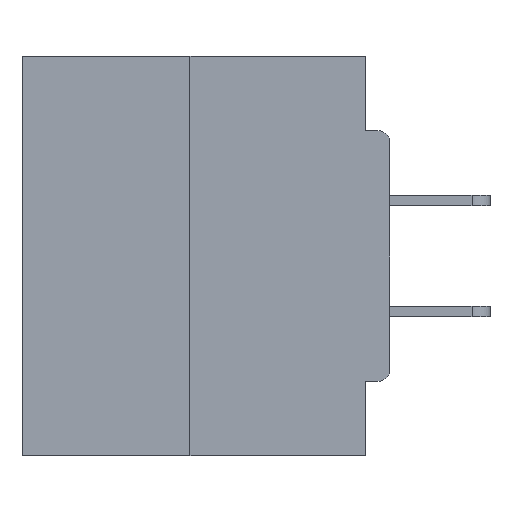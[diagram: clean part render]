
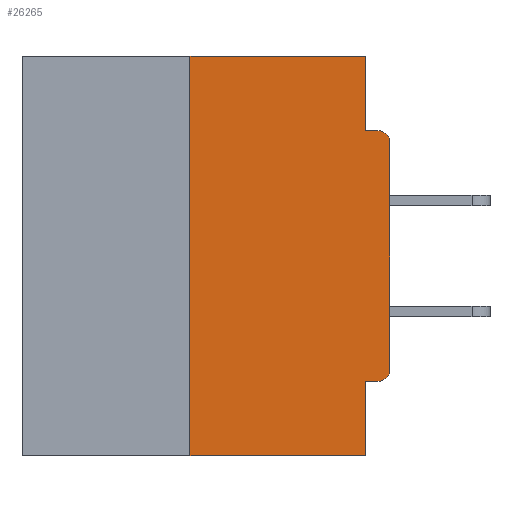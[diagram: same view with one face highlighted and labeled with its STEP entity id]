
A CAD part, left-side view. The second image highlights one B-rep face of the part: STEP entity #26265.
In plain terms, the highlighted planar face has unit normal (-1, 0, 0).
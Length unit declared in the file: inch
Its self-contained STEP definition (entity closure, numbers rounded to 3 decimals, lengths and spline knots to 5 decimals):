
#875 = DIRECTION ( 'NONE',  ( 0., 1., 0. ) ) ;
#1346 = CARTESIAN_POINT ( 'NONE',  ( 0., 0.46, 0. ) ) ;
#1678 = CARTESIAN_POINT ( 'NONE',  ( 0., 0.031, 0. ) ) ;
#2072 = DIRECTION ( 'NONE',  ( 0., 0., -1. ) ) ;
#2079 = AXIS2_PLACEMENT_3D ( 'NONE', #20776, #26328, #14355 ) ;
#2173 = CARTESIAN_POINT ( 'NONE',  ( 0., 0.031, -0.0935 ) ) ;
#2442 = CIRCLE ( 'NONE', #2079, 0.015 ) ;
#2732 = ORIENTED_EDGE ( 'NONE', *, *, #28134, .T. ) ;
#3569 = LINE ( 'NONE', #17001, #16551 ) ;
#4416 = VERTEX_POINT ( 'NONE', #1678 ) ;
#4546 = FACE_OUTER_BOUND ( 'NONE', #31437, .T. ) ;
#4741 = ORIENTED_EDGE ( 'NONE', *, *, #11772, .T. ) ;
#5494 = AXIS2_PLACEMENT_3D ( 'NONE', #18120, #24170, #39622 ) ;
#5855 = CARTESIAN_POINT ( 'NONE',  ( 0., 0., 0. ) ) ;
#6552 = LINE ( 'NONE', #32790, #29176 ) ;
#7020 = VECTOR ( 'NONE', #16874, 39.37008 ) ;
#7165 = CARTESIAN_POINT ( 'NONE',  ( 0., 0.25, 0. ) ) ;
#7606 = EDGE_CURVE ( 'NONE', #38162, #8715, #23775, .T. ) ;
#7782 = CARTESIAN_POINT ( 'NONE',  ( 0., 0.015, -0.0935 ) ) ;
#8039 = DIRECTION ( 'NONE',  ( 0., -1., 0. ) ) ;
#8715 = VERTEX_POINT ( 'NONE', #27837 ) ;
#8838 = ORIENTED_EDGE ( 'NONE', *, *, #26381, .F. ) ;
#9383 = ORIENTED_EDGE ( 'NONE', *, *, #21197, .T. ) ;
#10501 = ORIENTED_EDGE ( 'NONE', *, *, #39046, .F. ) ;
#11159 = VERTEX_POINT ( 'NONE', #16695 ) ;
#11772 = EDGE_CURVE ( 'NONE', #11159, #28743, #6552, .T. ) ;
#13876 = PLANE ( 'NONE',  #21875 ) ;
#13897 = CARTESIAN_POINT ( 'NONE',  ( 0., 0., -0.1085 ) ) ;
#14192 = CARTESIAN_POINT ( 'NONE',  ( 0., 0., -0.3915 ) ) ;
#14355 = DIRECTION ( 'NONE',  ( 0., 0., -1. ) ) ;
#15126 = EDGE_CURVE ( 'NONE', #16655, #4416, #16338, .T. ) ;
#16338 = LINE ( 'NONE', #36605, #36119 ) ;
#16551 = VECTOR ( 'NONE', #2072, 39.37008 ) ;
#16650 = DIRECTION ( 'NONE',  ( 1., 0., 0. ) ) ;
#16655 = VERTEX_POINT ( 'NONE', #23338 ) ;
#16695 = CARTESIAN_POINT ( 'NONE',  ( 0., 0.25, -0.5 ) ) ;
#16832 = ORIENTED_EDGE ( 'NONE', *, *, #23366, .F. ) ;
#16874 = DIRECTION ( 'NONE',  ( 0., 0., -1. ) ) ;
#16960 = VERTEX_POINT ( 'NONE', #13897 ) ;
#17001 = CARTESIAN_POINT ( 'NONE',  ( 0., 0.031, -0.5 ) ) ;
#17067 = DIRECTION ( 'NONE',  ( 0., 0., -1. ) ) ;
#17168 = ORIENTED_EDGE ( 'NONE', *, *, #15126, .F. ) ;
#18120 = CARTESIAN_POINT ( 'NONE',  ( 0., 0.015, -0.1085 ) ) ;
#20385 = CIRCLE ( 'NONE', #5494, 0.015 ) ;
#20776 = CARTESIAN_POINT ( 'NONE',  ( 0., 0.015, -0.3915 ) ) ;
#21197 = EDGE_CURVE ( 'NONE', #21769, #16960, #25792, .T. ) ;
#21636 = ORIENTED_EDGE ( 'NONE', *, *, #25235, .F. ) ;
#21769 = VERTEX_POINT ( 'NONE', #14192 ) ;
#21875 = AXIS2_PLACEMENT_3D ( 'NONE', #1346, #16650, #17067 ) ;
#22458 = CARTESIAN_POINT ( 'NONE',  ( 0., 0.015, -0.4065 ) ) ;
#22935 = CARTESIAN_POINT ( 'NONE',  ( 0., 0., -0.4065 ) ) ;
#23095 = VECTOR ( 'NONE', #28563, 39.37008 ) ;
#23338 = CARTESIAN_POINT ( 'NONE',  ( 0., 0.25, 0. ) ) ;
#23366 = EDGE_CURVE ( 'NONE', #11159, #16655, #39444, .T. ) ;
#23775 = LINE ( 'NONE', #22935, #32000 ) ;
#24170 = DIRECTION ( 'NONE',  ( -1., 0., 0. ) ) ;
#24762 = VECTOR ( 'NONE', #39376, 39.37008 ) ;
#25235 = EDGE_CURVE ( 'NONE', #4416, #25847, #38786, .T. ) ;
#25792 = LINE ( 'NONE', #5855, #35900 ) ;
#25847 = VERTEX_POINT ( 'NONE', #2173 ) ;
#26199 = LINE ( 'NONE', #36189, #24762 ) ;
#26240 = CARTESIAN_POINT ( 'NONE',  ( 0., 0.031, -0.5 ) ) ;
#26265 = ADVANCED_FACE ( 'NONE', ( #4546 ), #13876, .F. ) ;
#26328 = DIRECTION ( 'NONE',  ( -1., 0., 0. ) ) ;
#26381 = EDGE_CURVE ( 'NONE', #25847, #36324, #26199, .T. ) ;
#27837 = CARTESIAN_POINT ( 'NONE',  ( 0., 0.031, -0.4065 ) ) ;
#28134 = EDGE_CURVE ( 'NONE', #38162, #21769, #2442, .T. ) ;
#28563 = DIRECTION ( 'NONE',  ( 0., 0., 1. ) ) ;
#28647 = ORIENTED_EDGE ( 'NONE', *, *, #7606, .F. ) ;
#28743 = VERTEX_POINT ( 'NONE', #26240 ) ;
#29176 = VECTOR ( 'NONE', #8039, 39.37008 ) ;
#30739 = EDGE_CURVE ( 'NONE', #16960, #36324, #20385, .T. ) ;
#31437 = EDGE_LOOP ( 'NONE', ( #17168, #16832, #4741, #10501, #28647, #2732, #9383, #35111, #8838, #21636 ) ) ;
#32000 = VECTOR ( 'NONE', #875, 39.37008 ) ;
#32790 = CARTESIAN_POINT ( 'NONE',  ( 0., 0.46, -0.5 ) ) ;
#35111 = ORIENTED_EDGE ( 'NONE', *, *, #30739, .T. ) ;
#35320 = CARTESIAN_POINT ( 'NONE',  ( 0., 0.031, 0. ) ) ;
#35900 = VECTOR ( 'NONE', #39474, 39.37008 ) ;
#36119 = VECTOR ( 'NONE', #36217, 39.37008 ) ;
#36189 = CARTESIAN_POINT ( 'NONE',  ( 0., 0., -0.0935 ) ) ;
#36217 = DIRECTION ( 'NONE',  ( 0., -1., 0. ) ) ;
#36324 = VERTEX_POINT ( 'NONE', #7782 ) ;
#36605 = CARTESIAN_POINT ( 'NONE',  ( 0., 0.46, 0. ) ) ;
#38162 = VERTEX_POINT ( 'NONE', #22458 ) ;
#38786 = LINE ( 'NONE', #35320, #7020 ) ;
#39046 = EDGE_CURVE ( 'NONE', #8715, #28743, #3569, .T. ) ;
#39376 = DIRECTION ( 'NONE',  ( 0., -1., 0. ) ) ;
#39444 = LINE ( 'NONE', #7165, #23095 ) ;
#39474 = DIRECTION ( 'NONE',  ( 0., 0., 1. ) ) ;
#39622 = DIRECTION ( 'NONE',  ( 0., 0., -1. ) ) ;
